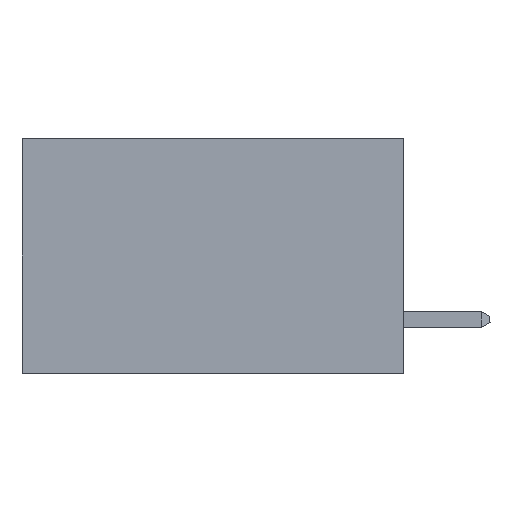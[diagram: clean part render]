
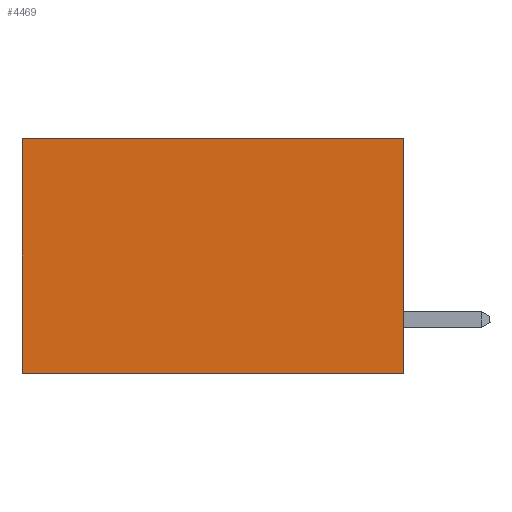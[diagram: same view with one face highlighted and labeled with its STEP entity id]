
A CAD part, left-side view. The second image highlights one B-rep face of the part: STEP entity #4469.
In plain terms, the highlighted planar face has unit normal (-1, 0, 0).
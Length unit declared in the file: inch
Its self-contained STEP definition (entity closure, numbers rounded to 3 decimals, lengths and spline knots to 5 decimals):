
#105 = CARTESIAN_POINT ( 'NONE',  ( 0.2875, 0., 0. ) ) ;
#128 = EDGE_CURVE ( 'NONE', #9500, #3198, #1860, .T. ) ;
#411 = CARTESIAN_POINT ( 'NONE',  ( 0.2875, 0., 0. ) ) ;
#524 = CARTESIAN_POINT ( 'NONE',  ( 0.2875, 0.6, 0. ) ) ;
#797 = CARTESIAN_POINT ( 'NONE',  ( 0.2875, 0., 0. ) ) ;
#906 = VECTOR ( 'NONE', #12013, 39.37008 ) ;
#1676 = VECTOR ( 'NONE', #3767, 39.37008 ) ;
#1860 = LINE ( 'NONE', #105, #2966 ) ;
#2579 = PLANE ( 'NONE',  #12409 ) ;
#2966 = VECTOR ( 'NONE', #5199, 39.37008 ) ;
#3093 = ORIENTED_EDGE ( 'NONE', *, *, #12281, .T. ) ;
#3188 = EDGE_LOOP ( 'NONE', ( #12124, #4911, #4272, #3093 ) ) ;
#3198 = VERTEX_POINT ( 'NONE', #7793 ) ;
#3486 = VERTEX_POINT ( 'NONE', #13226 ) ;
#3758 = VECTOR ( 'NONE', #9509, 39.37008 ) ;
#3767 = DIRECTION ( 'NONE',  ( 0., 0., -1. ) ) ;
#3826 = CARTESIAN_POINT ( 'NONE',  ( 0.2875, 0., -0.37 ) ) ;
#4272 = ORIENTED_EDGE ( 'NONE', *, *, #128, .F. ) ;
#4469 = ADVANCED_FACE ( 'NONE', ( #12684 ), #2579, .F. ) ;
#4911 = ORIENTED_EDGE ( 'NONE', *, *, #5163, .F. ) ;
#5163 = EDGE_CURVE ( 'NONE', #3198, #3486, #11050, .T. ) ;
#5199 = DIRECTION ( 'NONE',  ( 0., 0., -1. ) ) ;
#7402 = EDGE_CURVE ( 'NONE', #9023, #3486, #10859, .T. ) ;
#7659 = DIRECTION ( 'NONE',  ( 1., 0., 0. ) ) ;
#7768 = DIRECTION ( 'NONE',  ( 0., 0., -1. ) ) ;
#7793 = CARTESIAN_POINT ( 'NONE',  ( 0.2875, 0., -0.37 ) ) ;
#9023 = VERTEX_POINT ( 'NONE', #9791 ) ;
#9500 = VERTEX_POINT ( 'NONE', #797 ) ;
#9509 = DIRECTION ( 'NONE',  ( 0., 1., 0. ) ) ;
#9791 = CARTESIAN_POINT ( 'NONE',  ( 0.2875, 0.6, 0. ) ) ;
#10492 = CARTESIAN_POINT ( 'NONE',  ( 0.2875, 0., 0. ) ) ;
#10851 = LINE ( 'NONE', #10492, #3758 ) ;
#10859 = LINE ( 'NONE', #524, #1676 ) ;
#11050 = LINE ( 'NONE', #3826, #906 ) ;
#12013 = DIRECTION ( 'NONE',  ( 0., 1., 0. ) ) ;
#12124 = ORIENTED_EDGE ( 'NONE', *, *, #7402, .T. ) ;
#12281 = EDGE_CURVE ( 'NONE', #9500, #9023, #10851, .T. ) ;
#12409 = AXIS2_PLACEMENT_3D ( 'NONE', #411, #7659, #7768 ) ;
#12684 = FACE_OUTER_BOUND ( 'NONE', #3188, .T. ) ;
#13226 = CARTESIAN_POINT ( 'NONE',  ( 0.2875, 0.6, -0.37 ) ) ;
